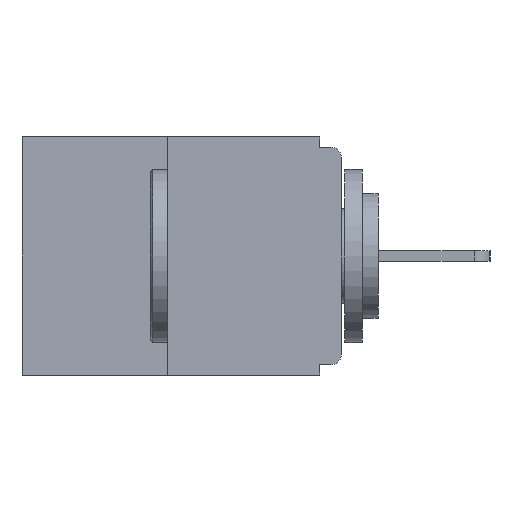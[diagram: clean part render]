
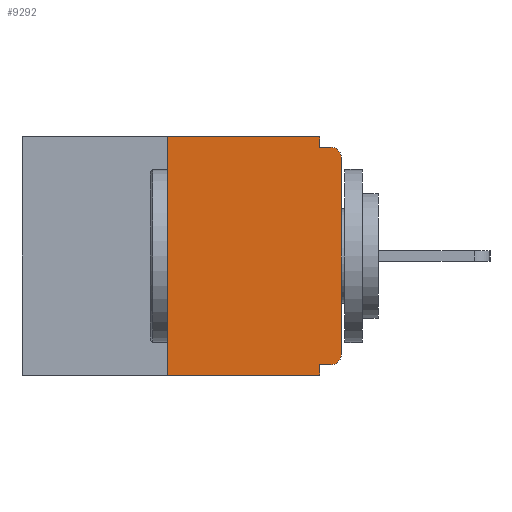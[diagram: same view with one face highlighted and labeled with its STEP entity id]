
A CAD part, left-side view. The second image highlights one B-rep face of the part: STEP entity #9292.
In plain terms, the highlighted planar face has unit normal (-1, 0, 0).
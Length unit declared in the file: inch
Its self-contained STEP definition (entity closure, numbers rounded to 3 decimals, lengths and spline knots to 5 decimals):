
#163 = AXIS2_PLACEMENT_3D ( 'NONE', #10902, #19199, #15723 ) ;
#319 = CARTESIAN_POINT ( 'NONE',  ( 0., 0.46, 0. ) ) ;
#474 = VERTEX_POINT ( 'NONE', #11287 ) ;
#591 = VECTOR ( 'NONE', #20017, 39.37008 ) ;
#653 = LINE ( 'NONE', #7115, #591 ) ;
#656 = ORIENTED_EDGE ( 'NONE', *, *, #1514, .F. ) ;
#913 = CARTESIAN_POINT ( 'NONE',  ( 0., 0., -0.313 ) ) ;
#1514 = EDGE_CURVE ( 'NONE', #474, #3329, #9235, .T. ) ;
#2815 = DIRECTION ( 'NONE',  ( 0., 0., 1. ) ) ;
#3286 = VERTEX_POINT ( 'NONE', #3456 ) ;
#3329 = VERTEX_POINT ( 'NONE', #13633 ) ;
#3456 = CARTESIAN_POINT ( 'NONE',  ( 0., 0.015, -0.015 ) ) ;
#3779 = VERTEX_POINT ( 'NONE', #18529 ) ;
#4045 = DIRECTION ( 'NONE',  ( 0., 1., 0. ) ) ;
#4278 = CARTESIAN_POINT ( 'NONE',  ( 0., 0.031, -0.015 ) ) ;
#4299 = LINE ( 'NONE', #7791, #16729 ) ;
#4767 = PLANE ( 'NONE',  #15423 ) ;
#4904 = LINE ( 'NONE', #6707, #15678 ) ;
#4959 = EDGE_CURVE ( 'NONE', #7313, #7691, #5699, .T. ) ;
#5031 = DIRECTION ( 'NONE',  ( 0., 0., -1. ) ) ;
#5361 = AXIS2_PLACEMENT_3D ( 'NONE', #18277, #20292, #5377 ) ;
#5377 = DIRECTION ( 'NONE',  ( 0., 0., -1. ) ) ;
#5479 = ORIENTED_EDGE ( 'NONE', *, *, #6688, .F. ) ;
#5699 = CIRCLE ( 'NONE', #5361, 0.015 ) ;
#5726 = CARTESIAN_POINT ( 'NONE',  ( 0., 0.015, -0.328 ) ) ;
#5946 = LINE ( 'NONE', #12444, #14552 ) ;
#6002 = ORIENTED_EDGE ( 'NONE', *, *, #18516, .F. ) ;
#6113 = EDGE_LOOP ( 'NONE', ( #656, #5479, #18912, #9745, #6002, #17930, #10630, #8957, #17299, #20506 ) ) ;
#6399 = EDGE_CURVE ( 'NONE', #3329, #8350, #11556, .T. ) ;
#6428 = CARTESIAN_POINT ( 'NONE',  ( 0., 0.46, 0. ) ) ;
#6688 = EDGE_CURVE ( 'NONE', #3779, #474, #4299, .T. ) ;
#6707 = CARTESIAN_POINT ( 'NONE',  ( 0., 0., -0.015 ) ) ;
#6727 = EDGE_CURVE ( 'NONE', #13717, #3286, #18404, .T. ) ;
#6728 = VERTEX_POINT ( 'NONE', #14268 ) ;
#6829 = EDGE_CURVE ( 'NONE', #8350, #3286, #4904, .T. ) ;
#7115 = CARTESIAN_POINT ( 'NONE',  ( 0., 0.46, -0.343 ) ) ;
#7313 = VERTEX_POINT ( 'NONE', #5726 ) ;
#7396 = LINE ( 'NONE', #13775, #13978 ) ;
#7602 = VECTOR ( 'NONE', #5031, 39.37008 ) ;
#7691 = VERTEX_POINT ( 'NONE', #913 ) ;
#7791 = CARTESIAN_POINT ( 'NONE',  ( 0., 0.25, 0. ) ) ;
#8350 = VERTEX_POINT ( 'NONE', #4278 ) ;
#8691 = VECTOR ( 'NONE', #15131, 39.37008 ) ;
#8957 = ORIENTED_EDGE ( 'NONE', *, *, #6727, .T. ) ;
#9235 = LINE ( 'NONE', #6428, #16822 ) ;
#9292 = ADVANCED_FACE ( 'NONE', ( #13068 ), #4767, .F. ) ;
#9369 = EDGE_CURVE ( 'NONE', #7691, #13717, #10220, .T. ) ;
#9745 = ORIENTED_EDGE ( 'NONE', *, *, #16878, .F. ) ;
#9911 = DIRECTION ( 'NONE',  ( 0., 0., -1. ) ) ;
#10220 = LINE ( 'NONE', #10648, #8691 ) ;
#10630 = ORIENTED_EDGE ( 'NONE', *, *, #9369, .T. ) ;
#10648 = CARTESIAN_POINT ( 'NONE',  ( 0., 0., 0. ) ) ;
#10744 = EDGE_CURVE ( 'NONE', #3779, #20145, #653, .T. ) ;
#10902 = CARTESIAN_POINT ( 'NONE',  ( 0., 0.015, -0.03 ) ) ;
#11287 = CARTESIAN_POINT ( 'NONE',  ( 0., 0.25, 0. ) ) ;
#11556 = LINE ( 'NONE', #19433, #7602 ) ;
#12444 = CARTESIAN_POINT ( 'NONE',  ( 0., 0., -0.328 ) ) ;
#13068 = FACE_OUTER_BOUND ( 'NONE', #6113, .T. ) ;
#13633 = CARTESIAN_POINT ( 'NONE',  ( 0., 0.031, 0. ) ) ;
#13717 = VERTEX_POINT ( 'NONE', #19164 ) ;
#13775 = CARTESIAN_POINT ( 'NONE',  ( 0., 0.031, -0.343 ) ) ;
#13978 = VECTOR ( 'NONE', #20187, 39.37008 ) ;
#14268 = CARTESIAN_POINT ( 'NONE',  ( 0., 0.031, -0.328 ) ) ;
#14552 = VECTOR ( 'NONE', #4045, 39.37008 ) ;
#14758 = DIRECTION ( 'NONE',  ( 0., -1., 0. ) ) ;
#15131 = DIRECTION ( 'NONE',  ( 0., 0., 1. ) ) ;
#15423 = AXIS2_PLACEMENT_3D ( 'NONE', #319, #19683, #9911 ) ;
#15449 = CARTESIAN_POINT ( 'NONE',  ( 0., 0.031, -0.343 ) ) ;
#15678 = VECTOR ( 'NONE', #14758, 39.37008 ) ;
#15723 = DIRECTION ( 'NONE',  ( 0., 0., -1. ) ) ;
#15856 = DIRECTION ( 'NONE',  ( 0., -1., 0. ) ) ;
#16729 = VECTOR ( 'NONE', #2815, 39.37008 ) ;
#16822 = VECTOR ( 'NONE', #15856, 39.37008 ) ;
#16878 = EDGE_CURVE ( 'NONE', #6728, #20145, #7396, .T. ) ;
#17299 = ORIENTED_EDGE ( 'NONE', *, *, #6829, .F. ) ;
#17930 = ORIENTED_EDGE ( 'NONE', *, *, #4959, .T. ) ;
#18277 = CARTESIAN_POINT ( 'NONE',  ( 0., 0.015, -0.313 ) ) ;
#18404 = CIRCLE ( 'NONE', #163, 0.015 ) ;
#18516 = EDGE_CURVE ( 'NONE', #7313, #6728, #5946, .T. ) ;
#18529 = CARTESIAN_POINT ( 'NONE',  ( 0., 0.25, -0.343 ) ) ;
#18912 = ORIENTED_EDGE ( 'NONE', *, *, #10744, .T. ) ;
#19164 = CARTESIAN_POINT ( 'NONE',  ( 0., 0., -0.03 ) ) ;
#19199 = DIRECTION ( 'NONE',  ( -1., 0., 0. ) ) ;
#19433 = CARTESIAN_POINT ( 'NONE',  ( 0., 0.031, 0. ) ) ;
#19683 = DIRECTION ( 'NONE',  ( 1., 0., 0. ) ) ;
#20017 = DIRECTION ( 'NONE',  ( 0., -1., 0. ) ) ;
#20145 = VERTEX_POINT ( 'NONE', #15449 ) ;
#20187 = DIRECTION ( 'NONE',  ( 0., 0., -1. ) ) ;
#20292 = DIRECTION ( 'NONE',  ( -1., 0., 0. ) ) ;
#20506 = ORIENTED_EDGE ( 'NONE', *, *, #6399, .F. ) ;
